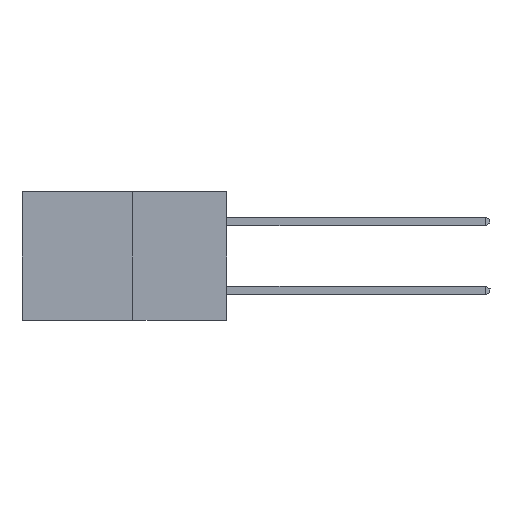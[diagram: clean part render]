
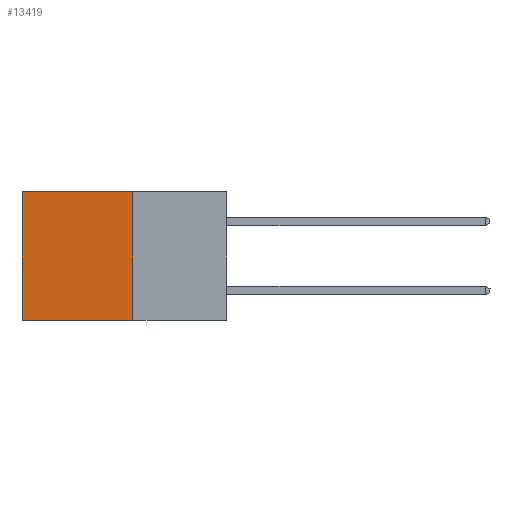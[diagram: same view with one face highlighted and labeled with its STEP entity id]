
A CAD part, left-side view. The second image highlights one B-rep face of the part: STEP entity #13419.
In plain terms, the highlighted planar face has unit normal (-1, 0, 0).
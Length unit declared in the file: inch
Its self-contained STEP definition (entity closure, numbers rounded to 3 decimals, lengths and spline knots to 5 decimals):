
#28 = VECTOR ( 'NONE', #10971, 39.37008 ) ;
#892 = CARTESIAN_POINT ( 'NONE',  ( 0.277, 0.59, 0. ) ) ;
#2495 = LINE ( 'NONE', #9224, #19971 ) ;
#2626 = EDGE_CURVE ( 'NONE', #13194, #27920, #2495, .T. ) ;
#3286 = CARTESIAN_POINT ( 'NONE',  ( 0.277, 0.59, -0.37 ) ) ;
#4168 = LINE ( 'NONE', #5798, #9509 ) ;
#4631 = EDGE_LOOP ( 'NONE', ( #25317, #10764, #6456, #26915 ) ) ;
#5798 = CARTESIAN_POINT ( 'NONE',  ( 0.277, 0.59, -0.37 ) ) ;
#6456 = ORIENTED_EDGE ( 'NONE', *, *, #13645, .F. ) ;
#9224 = CARTESIAN_POINT ( 'NONE',  ( 0.277, 0.27, 0. ) ) ;
#9506 = DIRECTION ( 'NONE',  ( 0., 1., 0. ) ) ;
#9509 = VECTOR ( 'NONE', #17183, 39.37008 ) ;
#10764 = ORIENTED_EDGE ( 'NONE', *, *, #14116, .F. ) ;
#10971 = DIRECTION ( 'NONE',  ( 0., 0., -1. ) ) ;
#11468 = VECTOR ( 'NONE', #16866, 39.37008 ) ;
#11493 = LINE ( 'NONE', #24484, #28 ) ;
#12567 = DIRECTION ( 'NONE',  ( 1., 0., 0. ) ) ;
#13010 = AXIS2_PLACEMENT_3D ( 'NONE', #26079, #12567, #28289 ) ;
#13194 = VERTEX_POINT ( 'NONE', #16298 ) ;
#13419 = ADVANCED_FACE ( 'NONE', ( #23182 ), #21479, .F. ) ;
#13645 = EDGE_CURVE ( 'NONE', #13194, #22838, #11493, .T. ) ;
#14116 = EDGE_CURVE ( 'NONE', #22838, #17241, #18192, .T. ) ;
#14578 = CARTESIAN_POINT ( 'NONE',  ( 0.277, 0.27, -0.37 ) ) ;
#16298 = CARTESIAN_POINT ( 'NONE',  ( 0.277, 0.27, 0. ) ) ;
#16866 = DIRECTION ( 'NONE',  ( 0., 1., 0. ) ) ;
#17183 = DIRECTION ( 'NONE',  ( 0., 0., -1. ) ) ;
#17241 = VERTEX_POINT ( 'NONE', #3286 ) ;
#18192 = LINE ( 'NONE', #14578, #11468 ) ;
#19971 = VECTOR ( 'NONE', #9506, 39.37008 ) ;
#21381 = EDGE_CURVE ( 'NONE', #27920, #17241, #4168, .T. ) ;
#21479 = PLANE ( 'NONE',  #13010 ) ;
#22838 = VERTEX_POINT ( 'NONE', #22900 ) ;
#22900 = CARTESIAN_POINT ( 'NONE',  ( 0.277, 0.27, -0.37 ) ) ;
#23182 = FACE_OUTER_BOUND ( 'NONE', #4631, .T. ) ;
#24484 = CARTESIAN_POINT ( 'NONE',  ( 0.277, 0.27, -0.37 ) ) ;
#25317 = ORIENTED_EDGE ( 'NONE', *, *, #21381, .T. ) ;
#26079 = CARTESIAN_POINT ( 'NONE',  ( 0.277, 0.27, -0.37 ) ) ;
#26915 = ORIENTED_EDGE ( 'NONE', *, *, #2626, .T. ) ;
#27920 = VERTEX_POINT ( 'NONE', #892 ) ;
#28289 = DIRECTION ( 'NONE',  ( 0., 0., -1. ) ) ;
